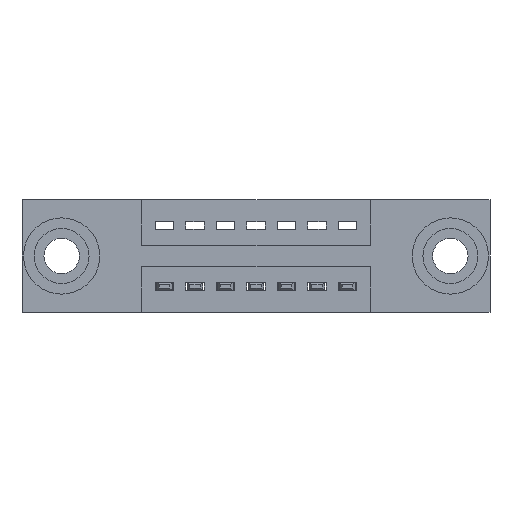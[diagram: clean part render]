
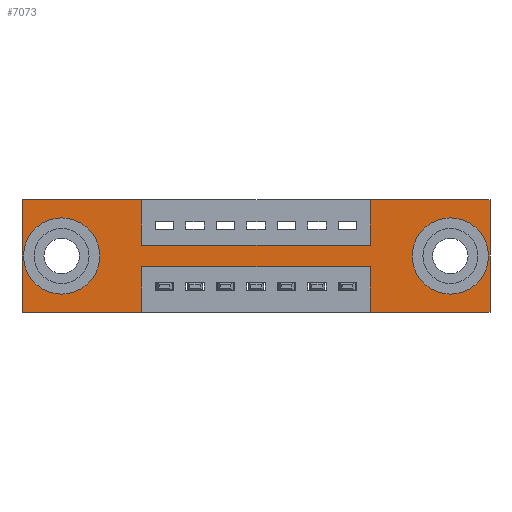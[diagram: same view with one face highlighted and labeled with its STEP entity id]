
A CAD part, front view. The second image highlights one B-rep face of the part: STEP entity #7073.
In plain terms, the highlighted planar face has unit normal (0, -1, 0).
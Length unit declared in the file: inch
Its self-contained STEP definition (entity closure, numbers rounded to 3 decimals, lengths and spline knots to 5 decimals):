
#60 = DIRECTION ( 'NONE',  ( 0., 0., -1. ) ) ;
#65 = FACE_BOUND ( 'NONE', #3047, .T. ) ;
#172 = CIRCLE ( 'NONE', #1869, 0.078 ) ;
#220 = CARTESIAN_POINT ( 'NONE',  ( 1.1425, 0., -0.37 ) ) ;
#236 = LINE ( 'NONE', #8420, #4070 ) ;
#277 = VECTOR ( 'NONE', #7055, 39.37008 ) ;
#374 = DIRECTION ( 'NONE',  ( 1., 0., 0. ) ) ;
#478 = DIRECTION ( 'NONE',  ( 0., 0., -1. ) ) ;
#536 = VECTOR ( 'NONE', #6985, 39.37008 ) ;
#594 = VERTEX_POINT ( 'NONE', #4243 ) ;
#619 = EDGE_LOOP ( 'NONE', ( #7385, #6621 ) ) ;
#845 = LINE ( 'NONE', #4644, #4742 ) ;
#897 = EDGE_CURVE ( 'NONE', #6872, #5058, #1456, .T. ) ;
#969 = CARTESIAN_POINT ( 'NONE',  ( 0.13, 0., -0.185 ) ) ;
#1076 = VERTEX_POINT ( 'NONE', #4790 ) ;
#1227 = CIRCLE ( 'NONE', #9849, 0.078 ) ;
#1252 = ORIENTED_EDGE ( 'NONE', *, *, #9929, .F. ) ;
#1342 = FACE_OUTER_BOUND ( 'NONE', #3422, .T. ) ;
#1456 = LINE ( 'NONE', #2246, #3390 ) ;
#1466 = DIRECTION ( 'NONE',  ( -1., 0., 0. ) ) ;
#1467 = EDGE_CURVE ( 'NONE', #4616, #2027, #3246, .T. ) ;
#1535 = DIRECTION ( 'NONE',  ( 0., 0., -1. ) ) ;
#1636 = EDGE_CURVE ( 'NONE', #2027, #3431, #9211, .T. ) ;
#1695 = CARTESIAN_POINT ( 'NONE',  ( 1.405, 0., -0.185 ) ) ;
#1739 = CARTESIAN_POINT ( 'NONE',  ( 1.535, 0., 0. ) ) ;
#1752 = ORIENTED_EDGE ( 'NONE', *, *, #897, .F. ) ;
#1792 = EDGE_CURVE ( 'NONE', #5142, #7338, #9966, .T. ) ;
#1869 = AXIS2_PLACEMENT_3D ( 'NONE', #1695, #3698, #478 ) ;
#1913 = CARTESIAN_POINT ( 'NONE',  ( 1.1425, 0., 0. ) ) ;
#2027 = VERTEX_POINT ( 'NONE', #10311 ) ;
#2033 = ORIENTED_EDGE ( 'NONE', *, *, #10041, .F. ) ;
#2058 = DIRECTION ( 'NONE',  ( 0., 1., 0. ) ) ;
#2161 = CARTESIAN_POINT ( 'NONE',  ( 1.1425, 0., -0.15 ) ) ;
#2183 = LINE ( 'NONE', #1913, #4959 ) ;
#2246 = CARTESIAN_POINT ( 'NONE',  ( 0., 0., 0. ) ) ;
#2500 = FACE_BOUND ( 'NONE', #619, .T. ) ;
#2502 = VECTOR ( 'NONE', #60, 39.37008 ) ;
#2504 = VECTOR ( 'NONE', #7687, 39.37008 ) ;
#2527 = CARTESIAN_POINT ( 'NONE',  ( 1.1425, 0., -0.22 ) ) ;
#2933 = DIRECTION ( 'NONE',  ( 0., 0., -1. ) ) ;
#2971 = CIRCLE ( 'NONE', #4976, 0.078 ) ;
#3037 = VERTEX_POINT ( 'NONE', #3731 ) ;
#3047 = EDGE_LOOP ( 'NONE', ( #6279, #9082 ) ) ;
#3185 = EDGE_CURVE ( 'NONE', #9021, #9658, #5552, .T. ) ;
#3246 = LINE ( 'NONE', #5482, #536 ) ;
#3390 = VECTOR ( 'NONE', #7056, 39.37008 ) ;
#3422 = EDGE_LOOP ( 'NONE', ( #2033, #6877, #10227, #9732, #7309, #1752, #1252, #5029, #7792, #7148, #4158, #7544 ) ) ;
#3431 = VERTEX_POINT ( 'NONE', #9983 ) ;
#3454 = AXIS2_PLACEMENT_3D ( 'NONE', #5434, #6356, #1535 ) ;
#3668 = VECTOR ( 'NONE', #374, 39.37008 ) ;
#3698 = DIRECTION ( 'NONE',  ( 0., 1., 0. ) ) ;
#3731 = CARTESIAN_POINT ( 'NONE',  ( 1.535, 0., -0.37 ) ) ;
#3896 = EDGE_CURVE ( 'NONE', #7443, #1076, #236, .T. ) ;
#3959 = PLANE ( 'NONE',  #3454 ) ;
#4070 = VECTOR ( 'NONE', #4427, 39.37008 ) ;
#4097 = LINE ( 'NONE', #4515, #8221 ) ;
#4158 = ORIENTED_EDGE ( 'NONE', *, *, #6865, .F. ) ;
#4243 = CARTESIAN_POINT ( 'NONE',  ( 1.405, 0., -0.263 ) ) ;
#4406 = EDGE_CURVE ( 'NONE', #9658, #5326, #7288, .T. ) ;
#4412 = DIRECTION ( 'NONE',  ( 0., 0., 1. ) ) ;
#4427 = DIRECTION ( 'NONE',  ( -1., 0., 0. ) ) ;
#4515 = CARTESIAN_POINT ( 'NONE',  ( 0.3925, 0., -0.37 ) ) ;
#4545 = CARTESIAN_POINT ( 'NONE',  ( 0.13, 0., -0.263 ) ) ;
#4616 = VERTEX_POINT ( 'NONE', #8272 ) ;
#4644 = CARTESIAN_POINT ( 'NONE',  ( 0., 0., -0.37 ) ) ;
#4716 = CARTESIAN_POINT ( 'NONE',  ( 0.3925, 0., 0. ) ) ;
#4742 = VECTOR ( 'NONE', #8741, 39.37008 ) ;
#4790 = CARTESIAN_POINT ( 'NONE',  ( 0., 0., -0.37 ) ) ;
#4832 = VERTEX_POINT ( 'NONE', #6603 ) ;
#4877 = CARTESIAN_POINT ( 'NONE',  ( 0.3925, 0., -0.37 ) ) ;
#4959 = VECTOR ( 'NONE', #4412, 39.37008 ) ;
#4976 = AXIS2_PLACEMENT_3D ( 'NONE', #969, #5046, #6384 ) ;
#5029 = ORIENTED_EDGE ( 'NONE', *, *, #5855, .F. ) ;
#5046 = DIRECTION ( 'NONE',  ( 0., 1., 0. ) ) ;
#5058 = VERTEX_POINT ( 'NONE', #1739 ) ;
#5142 = VERTEX_POINT ( 'NONE', #8426 ) ;
#5219 = CARTESIAN_POINT ( 'NONE',  ( 0.3925, 0., -0.15 ) ) ;
#5326 = VERTEX_POINT ( 'NONE', #6527 ) ;
#5393 = EDGE_CURVE ( 'NONE', #5058, #3037, #9518, .T. ) ;
#5434 = CARTESIAN_POINT ( 'NONE',  ( 0., 0., -0.37 ) ) ;
#5482 = CARTESIAN_POINT ( 'NONE',  ( 0., 0., 0. ) ) ;
#5552 = LINE ( 'NONE', #8651, #6185 ) ;
#5793 = AXIS2_PLACEMENT_3D ( 'NONE', #6059, #2058, #9346 ) ;
#5855 = EDGE_CURVE ( 'NONE', #3431, #7169, #6769, .T. ) ;
#6059 = CARTESIAN_POINT ( 'NONE',  ( 0.13, 0., -0.185 ) ) ;
#6153 = DIRECTION ( 'NONE',  ( 0., 0., -1. ) ) ;
#6185 = VECTOR ( 'NONE', #8722, 39.37008 ) ;
#6216 = CARTESIAN_POINT ( 'NONE',  ( 1.1425, 0., 0. ) ) ;
#6279 = ORIENTED_EDGE ( 'NONE', *, *, #1792, .T. ) ;
#6356 = DIRECTION ( 'NONE',  ( 0., -1., 0. ) ) ;
#6384 = DIRECTION ( 'NONE',  ( 0., 0., 1. ) ) ;
#6527 = CARTESIAN_POINT ( 'NONE',  ( 0.3925, 0., -0.22 ) ) ;
#6603 = CARTESIAN_POINT ( 'NONE',  ( 1.405, 0., -0.107 ) ) ;
#6621 = ORIENTED_EDGE ( 'NONE', *, *, #8798, .T. ) ;
#6638 = CARTESIAN_POINT ( 'NONE',  ( 1.535, 0., 0. ) ) ;
#6769 = LINE ( 'NONE', #5219, #3668 ) ;
#6865 = EDGE_CURVE ( 'NONE', #1076, #4616, #7019, .T. ) ;
#6872 = VERTEX_POINT ( 'NONE', #6216 ) ;
#6877 = ORIENTED_EDGE ( 'NONE', *, *, #4406, .F. ) ;
#6886 = EDGE_CURVE ( 'NONE', #4832, #594, #1227, .T. ) ;
#6892 = CARTESIAN_POINT ( 'NONE',  ( 0., 0., 0. ) ) ;
#6919 = DIRECTION ( 'NONE',  ( 0., 1., 0. ) ) ;
#6985 = DIRECTION ( 'NONE',  ( 1., 0., 0. ) ) ;
#7019 = LINE ( 'NONE', #6892, #2504 ) ;
#7029 = VECTOR ( 'NONE', #1466, 39.37008 ) ;
#7055 = DIRECTION ( 'NONE',  ( 0., 0., -1. ) ) ;
#7056 = DIRECTION ( 'NONE',  ( 1., 0., 0. ) ) ;
#7073 = ADVANCED_FACE ( 'NONE', ( #2500, #65, #1342 ), #3959, .T. ) ;
#7148 = ORIENTED_EDGE ( 'NONE', *, *, #1467, .F. ) ;
#7169 = VERTEX_POINT ( 'NONE', #2161 ) ;
#7288 = LINE ( 'NONE', #8561, #7029 ) ;
#7309 = ORIENTED_EDGE ( 'NONE', *, *, #5393, .F. ) ;
#7338 = VERTEX_POINT ( 'NONE', #4545 ) ;
#7385 = ORIENTED_EDGE ( 'NONE', *, *, #6886, .T. ) ;
#7443 = VERTEX_POINT ( 'NONE', #4877 ) ;
#7544 = ORIENTED_EDGE ( 'NONE', *, *, #3896, .F. ) ;
#7687 = DIRECTION ( 'NONE',  ( 0., 0., 1. ) ) ;
#7792 = ORIENTED_EDGE ( 'NONE', *, *, #1636, .F. ) ;
#8221 = VECTOR ( 'NONE', #6153, 39.37008 ) ;
#8272 = CARTESIAN_POINT ( 'NONE',  ( 0., 0., 0. ) ) ;
#8420 = CARTESIAN_POINT ( 'NONE',  ( 0., 0., -0.37 ) ) ;
#8426 = CARTESIAN_POINT ( 'NONE',  ( 0.13, 0., -0.107 ) ) ;
#8439 = EDGE_CURVE ( 'NONE', #7338, #5142, #2971, .T. ) ;
#8542 = CARTESIAN_POINT ( 'NONE',  ( 1.405, 0., -0.185 ) ) ;
#8561 = CARTESIAN_POINT ( 'NONE',  ( 0.3925, 0., -0.22 ) ) ;
#8651 = CARTESIAN_POINT ( 'NONE',  ( 1.1425, 0., -0.37 ) ) ;
#8722 = DIRECTION ( 'NONE',  ( 0., 0., 1. ) ) ;
#8726 = EDGE_CURVE ( 'NONE', #3037, #9021, #845, .T. ) ;
#8741 = DIRECTION ( 'NONE',  ( -1., 0., 0. ) ) ;
#8798 = EDGE_CURVE ( 'NONE', #594, #4832, #172, .T. ) ;
#9021 = VERTEX_POINT ( 'NONE', #220 ) ;
#9082 = ORIENTED_EDGE ( 'NONE', *, *, #8439, .T. ) ;
#9211 = LINE ( 'NONE', #4716, #277 ) ;
#9346 = DIRECTION ( 'NONE',  ( 0., 0., 1. ) ) ;
#9518 = LINE ( 'NONE', #6638, #2502 ) ;
#9658 = VERTEX_POINT ( 'NONE', #2527 ) ;
#9732 = ORIENTED_EDGE ( 'NONE', *, *, #8726, .F. ) ;
#9849 = AXIS2_PLACEMENT_3D ( 'NONE', #8542, #6919, #2933 ) ;
#9929 = EDGE_CURVE ( 'NONE', #7169, #6872, #2183, .T. ) ;
#9966 = CIRCLE ( 'NONE', #5793, 0.078 ) ;
#9983 = CARTESIAN_POINT ( 'NONE',  ( 0.3925, 0., -0.15 ) ) ;
#10041 = EDGE_CURVE ( 'NONE', #5326, #7443, #4097, .T. ) ;
#10227 = ORIENTED_EDGE ( 'NONE', *, *, #3185, .F. ) ;
#10311 = CARTESIAN_POINT ( 'NONE',  ( 0.3925, 0., 0. ) ) ;
